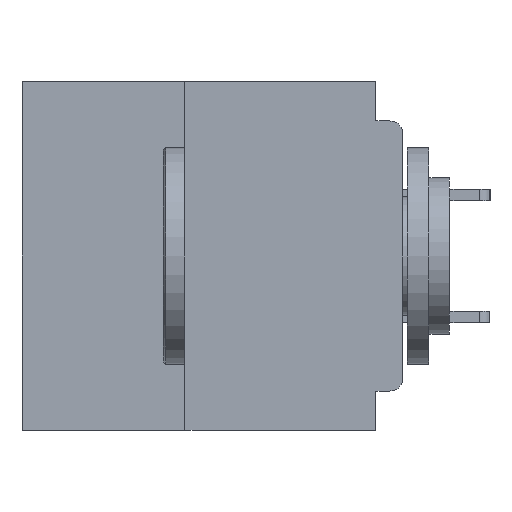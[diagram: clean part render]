
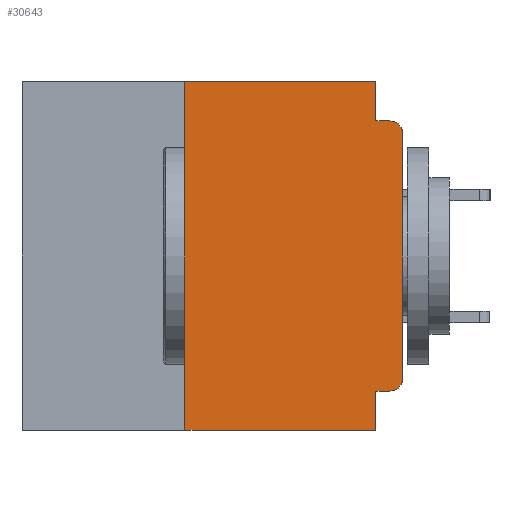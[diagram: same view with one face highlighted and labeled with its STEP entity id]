
A CAD part, left-side view. The second image highlights one B-rep face of the part: STEP entity #30643.
In plain terms, the highlighted planar face has unit normal (-1, 0, 0).
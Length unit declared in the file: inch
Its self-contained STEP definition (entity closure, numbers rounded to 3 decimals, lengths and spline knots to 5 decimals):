
#93 = EDGE_CURVE ( 'NONE', #50669, #18573, #10408, .T. ) ;
#564 = CARTESIAN_POINT ( 'NONE',  ( 0., 0., -0.045 ) ) ;
#717 = CARTESIAN_POINT ( 'NONE',  ( 0., 0.437, 0. ) ) ;
#1797 = ORIENTED_EDGE ( 'NONE', *, *, #23017, .F. ) ;
#2146 = EDGE_CURVE ( 'NONE', #23778, #18573, #9104, .T. ) ;
#2985 = ORIENTED_EDGE ( 'NONE', *, *, #38743, .F. ) ;
#4583 = VECTOR ( 'NONE', #48659, 39.37008 ) ;
#4983 = DIRECTION ( 'NONE',  ( 0., 0., -1. ) ) ;
#5528 = CARTESIAN_POINT ( 'NONE',  ( 0., 0.031, -0.045 ) ) ;
#6924 = CARTESIAN_POINT ( 'NONE',  ( 0., 0.031, 0. ) ) ;
#8142 = DIRECTION ( 'NONE',  ( 0., 0., -1. ) ) ;
#8232 = AXIS2_PLACEMENT_3D ( 'NONE', #717, #30123, #4983 ) ;
#8391 = VECTOR ( 'NONE', #44959, 39.37008 ) ;
#9092 = VECTOR ( 'NONE', #38954, 39.37008 ) ;
#9104 = CIRCLE ( 'NONE', #17198, 0.015 ) ;
#10282 = CARTESIAN_POINT ( 'NONE',  ( 0., 0.437, 0. ) ) ;
#10408 = LINE ( 'NONE', #564, #9092 ) ;
#10424 = AXIS2_PLACEMENT_3D ( 'NONE', #35619, #10604, #39804 ) ;
#10604 = DIRECTION ( 'NONE',  ( -1., 0., 0. ) ) ;
#10908 = CARTESIAN_POINT ( 'NONE',  ( 0., 0.015, -0.045 ) ) ;
#12021 = EDGE_CURVE ( 'NONE', #33776, #23778, #52267, .T. ) ;
#12534 = EDGE_CURVE ( 'NONE', #53344, #44743, #48314, .T. ) ;
#12827 = ORIENTED_EDGE ( 'NONE', *, *, #93, .F. ) ;
#13230 = PLANE ( 'NONE',  #8232 ) ;
#15001 = CARTESIAN_POINT ( 'NONE',  ( 0., 0.031, -0.4 ) ) ;
#15127 = CARTESIAN_POINT ( 'NONE',  ( 0., 0., 0. ) ) ;
#15130 = VECTOR ( 'NONE', #8142, 39.37008 ) ;
#15827 = CARTESIAN_POINT ( 'NONE',  ( 0., 0., -0.355 ) ) ;
#16410 = CARTESIAN_POINT ( 'NONE',  ( 0., 0.25, -0.4 ) ) ;
#17198 = AXIS2_PLACEMENT_3D ( 'NONE', #41799, #41661, #41556 ) ;
#17977 = CARTESIAN_POINT ( 'NONE',  ( 0., 0.25, 0. ) ) ;
#18063 = ORIENTED_EDGE ( 'NONE', *, *, #12021, .T. ) ;
#18573 = VERTEX_POINT ( 'NONE', #10908 ) ;
#19396 = ORIENTED_EDGE ( 'NONE', *, *, #2146, .T. ) ;
#19482 = VECTOR ( 'NONE', #36190, 39.37008 ) ;
#19699 = CARTESIAN_POINT ( 'NONE',  ( 0., 0.437, -0.4 ) ) ;
#21045 = EDGE_CURVE ( 'NONE', #34359, #46304, #36649, .T. ) ;
#21068 = CARTESIAN_POINT ( 'NONE',  ( 0., 0., -0.34 ) ) ;
#22189 = ORIENTED_EDGE ( 'NONE', *, *, #12534, .F. ) ;
#23017 = EDGE_CURVE ( 'NONE', #38270, #53344, #30683, .T. ) ;
#23778 = VERTEX_POINT ( 'NONE', #28973 ) ;
#24185 = VERTEX_POINT ( 'NONE', #25297 ) ;
#25297 = CARTESIAN_POINT ( 'NONE',  ( 0., 0.031, 0. ) ) ;
#28973 = CARTESIAN_POINT ( 'NONE',  ( 0., 0., -0.06 ) ) ;
#30123 = DIRECTION ( 'NONE',  ( 1., 0., 0. ) ) ;
#30643 = ADVANCED_FACE ( 'NONE', ( #53167 ), #13230, .F. ) ;
#30683 = LINE ( 'NONE', #15827, #8391 ) ;
#31982 = ORIENTED_EDGE ( 'NONE', *, *, #50390, .T. ) ;
#33115 = CARTESIAN_POINT ( 'NONE',  ( 0., 0.031, -0.355 ) ) ;
#33776 = VERTEX_POINT ( 'NONE', #21068 ) ;
#34359 = VERTEX_POINT ( 'NONE', #16410 ) ;
#35085 = ORIENTED_EDGE ( 'NONE', *, *, #37010, .F. ) ;
#35619 = CARTESIAN_POINT ( 'NONE',  ( 0., 0.015, -0.34 ) ) ;
#36190 = DIRECTION ( 'NONE',  ( 0., 0., -1. ) ) ;
#36455 = DIRECTION ( 'NONE',  ( 0., -1., 0. ) ) ;
#36649 = LINE ( 'NONE', #40581, #4583 ) ;
#36803 = CARTESIAN_POINT ( 'NONE',  ( 0., 0.015, -0.355 ) ) ;
#37010 = EDGE_CURVE ( 'NONE', #24185, #50669, #41626, .T. ) ;
#37337 = VECTOR ( 'NONE', #51757, 39.37008 ) ;
#38270 = VERTEX_POINT ( 'NONE', #36803 ) ;
#38743 = EDGE_CURVE ( 'NONE', #46304, #24185, #48305, .T. ) ;
#38954 = DIRECTION ( 'NONE',  ( 0., -1., 0. ) ) ;
#39043 = ORIENTED_EDGE ( 'NONE', *, *, #21045, .F. ) ;
#39762 = LINE ( 'NONE', #19699, #48109 ) ;
#39804 = DIRECTION ( 'NONE',  ( 0., 0., -1. ) ) ;
#40465 = ORIENTED_EDGE ( 'NONE', *, *, #41924, .T. ) ;
#40581 = CARTESIAN_POINT ( 'NONE',  ( 0., 0.25, -0.4 ) ) ;
#41303 = VECTOR ( 'NONE', #48397, 39.37008 ) ;
#41513 = CIRCLE ( 'NONE', #10424, 0.015 ) ;
#41556 = DIRECTION ( 'NONE',  ( 0., 0., -1. ) ) ;
#41626 = LINE ( 'NONE', #6924, #19482 ) ;
#41661 = DIRECTION ( 'NONE',  ( -1., 0., 0. ) ) ;
#41799 = CARTESIAN_POINT ( 'NONE',  ( 0., 0.015, -0.06 ) ) ;
#41924 = EDGE_CURVE ( 'NONE', #38270, #33776, #41513, .T. ) ;
#44743 = VERTEX_POINT ( 'NONE', #15001 ) ;
#44959 = DIRECTION ( 'NONE',  ( 0., 1., 0. ) ) ;
#46304 = VERTEX_POINT ( 'NONE', #17977 ) ;
#48109 = VECTOR ( 'NONE', #36455, 39.37008 ) ;
#48305 = LINE ( 'NONE', #10282, #37337 ) ;
#48314 = LINE ( 'NONE', #53809, #15130 ) ;
#48397 = DIRECTION ( 'NONE',  ( 0., 0., 1. ) ) ;
#48659 = DIRECTION ( 'NONE',  ( 0., 0., 1. ) ) ;
#50306 = EDGE_LOOP ( 'NONE', ( #18063, #19396, #12827, #35085, #2985, #39043, #31982, #22189, #1797, #40465 ) ) ;
#50390 = EDGE_CURVE ( 'NONE', #34359, #44743, #39762, .T. ) ;
#50669 = VERTEX_POINT ( 'NONE', #5528 ) ;
#51757 = DIRECTION ( 'NONE',  ( 0., -1., 0. ) ) ;
#52267 = LINE ( 'NONE', #15127, #41303 ) ;
#53167 = FACE_OUTER_BOUND ( 'NONE', #50306, .T. ) ;
#53344 = VERTEX_POINT ( 'NONE', #33115 ) ;
#53809 = CARTESIAN_POINT ( 'NONE',  ( 0., 0.031, -0.4 ) ) ;
